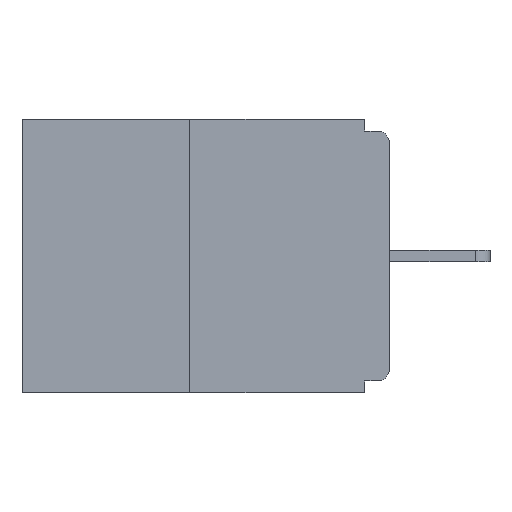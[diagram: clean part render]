
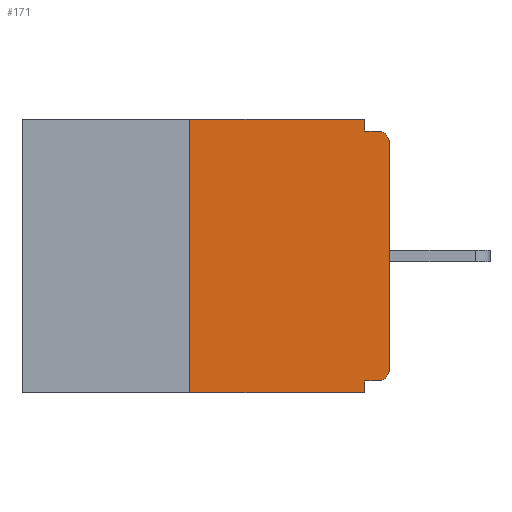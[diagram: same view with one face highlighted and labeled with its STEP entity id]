
A CAD part, left-side view. The second image highlights one B-rep face of the part: STEP entity #171.
In plain terms, the highlighted planar face has unit normal (-1, 0, 0).
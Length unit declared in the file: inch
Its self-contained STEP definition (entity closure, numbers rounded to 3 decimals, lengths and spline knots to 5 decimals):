
#47 = LINE ( 'NONE', #8881, #184 ) ;
#171 = ADVANCED_FACE ( 'NONE', ( #5599 ), #9420, .F. ) ;
#184 = VECTOR ( 'NONE', #10004, 39.37008 ) ;
#208 = EDGE_LOOP ( 'NONE', ( #5698, #8267, #6809, #2005, #5004, #4172, #3948, #3840, #4749, #7733 ) ) ;
#215 = CARTESIAN_POINT ( 'NONE',  ( 0., 0.46, -0.343 ) ) ;
#299 = VERTEX_POINT ( 'NONE', #7699 ) ;
#436 = AXIS2_PLACEMENT_3D ( 'NONE', #7407, #6733, #6550 ) ;
#534 = VECTOR ( 'NONE', #6665, 39.37008 ) ;
#879 = LINE ( 'NONE', #5942, #534 ) ;
#942 = CARTESIAN_POINT ( 'NONE',  ( 0., 0.031, -0.015 ) ) ;
#998 = VERTEX_POINT ( 'NONE', #942 ) ;
#1353 = EDGE_CURVE ( 'NONE', #2045, #8101, #3386, .T. ) ;
#1361 = CARTESIAN_POINT ( 'NONE',  ( 0., 0., -0.328 ) ) ;
#1407 = EDGE_CURVE ( 'NONE', #2045, #6537, #3336, .T. ) ;
#1527 = EDGE_CURVE ( 'NONE', #3534, #6537, #2998, .T. ) ;
#1554 = EDGE_CURVE ( 'NONE', #5897, #3534, #2892, .T. ) ;
#1609 = EDGE_CURVE ( 'NONE', #8135, #998, #2805, .T. ) ;
#2005 = ORIENTED_EDGE ( 'NONE', *, *, #1527, .F. ) ;
#2045 = VERTEX_POINT ( 'NONE', #5724 ) ;
#2105 = CARTESIAN_POINT ( 'NONE',  ( 0., 0., -0.015 ) ) ;
#2471 = EDGE_CURVE ( 'NONE', #8101, #8135, #47, .T. ) ;
#2760 = VECTOR ( 'NONE', #3348, 39.37008 ) ;
#2804 = DIRECTION ( 'NONE',  ( 0., 0., 1. ) ) ;
#2805 = LINE ( 'NONE', #10197, #2760 ) ;
#2863 = VECTOR ( 'NONE', #9930, 39.37008 ) ;
#2892 = LINE ( 'NONE', #1361, #2863 ) ;
#2925 = DIRECTION ( 'NONE',  ( 0., -1., 0. ) ) ;
#2951 = VECTOR ( 'NONE', #5788, 39.37008 ) ;
#2992 = CARTESIAN_POINT ( 'NONE',  ( 0., 0.25, 0. ) ) ;
#2998 = LINE ( 'NONE', #4763, #2951 ) ;
#3192 = AXIS2_PLACEMENT_3D ( 'NONE', #7427, #7318, #7304 ) ;
#3228 = VECTOR ( 'NONE', #2925, 39.37008 ) ;
#3336 = LINE ( 'NONE', #215, #3228 ) ;
#3348 = DIRECTION ( 'NONE',  ( 0., 0., -1. ) ) ;
#3366 = VECTOR ( 'NONE', #2804, 39.37008 ) ;
#3386 = LINE ( 'NONE', #2992, #3366 ) ;
#3403 = DIRECTION ( 'NONE',  ( -1., 0., 0. ) ) ;
#3534 = VERTEX_POINT ( 'NONE', #6160 ) ;
#3840 = ORIENTED_EDGE ( 'NONE', *, *, #5633, .T. ) ;
#3948 = ORIENTED_EDGE ( 'NONE', *, *, #9429, .T. ) ;
#3957 = CARTESIAN_POINT ( 'NONE',  ( 0., 0., -0.313 ) ) ;
#4172 = ORIENTED_EDGE ( 'NONE', *, *, #4719, .T. ) ;
#4719 = EDGE_CURVE ( 'NONE', #5897, #8591, #6618, .T. ) ;
#4749 = ORIENTED_EDGE ( 'NONE', *, *, #5171, .F. ) ;
#4763 = CARTESIAN_POINT ( 'NONE',  ( 0., 0.031, -0.343 ) ) ;
#5004 = ORIENTED_EDGE ( 'NONE', *, *, #1554, .F. ) ;
#5067 = DIRECTION ( 'NONE',  ( 0., -1., 0. ) ) ;
#5171 = EDGE_CURVE ( 'NONE', #998, #299, #7346, .T. ) ;
#5196 = VECTOR ( 'NONE', #5067, 39.37008 ) ;
#5599 = FACE_OUTER_BOUND ( 'NONE', #208, .T. ) ;
#5633 = EDGE_CURVE ( 'NONE', #8870, #299, #7892, .T. ) ;
#5698 = ORIENTED_EDGE ( 'NONE', *, *, #2471, .F. ) ;
#5724 = CARTESIAN_POINT ( 'NONE',  ( 0., 0.25, -0.343 ) ) ;
#5788 = DIRECTION ( 'NONE',  ( 0., 0., -1. ) ) ;
#5897 = VERTEX_POINT ( 'NONE', #9774 ) ;
#5942 = CARTESIAN_POINT ( 'NONE',  ( 0., 0., 0. ) ) ;
#6160 = CARTESIAN_POINT ( 'NONE',  ( 0., 0.031, -0.328 ) ) ;
#6537 = VERTEX_POINT ( 'NONE', #9851 ) ;
#6550 = DIRECTION ( 'NONE',  ( 0., 0., -1. ) ) ;
#6618 = CIRCLE ( 'NONE', #3192, 0.015 ) ;
#6665 = DIRECTION ( 'NONE',  ( 0., 0., 1. ) ) ;
#6733 = DIRECTION ( 'NONE',  ( 1., 0., 0. ) ) ;
#6809 = ORIENTED_EDGE ( 'NONE', *, *, #1407, .T. ) ;
#7304 = DIRECTION ( 'NONE',  ( 0., 0., -1. ) ) ;
#7318 = DIRECTION ( 'NONE',  ( -1., 0., 0. ) ) ;
#7346 = LINE ( 'NONE', #2105, #5196 ) ;
#7407 = CARTESIAN_POINT ( 'NONE',  ( 0., 0.46, 0. ) ) ;
#7427 = CARTESIAN_POINT ( 'NONE',  ( 0., 0.015, -0.313 ) ) ;
#7699 = CARTESIAN_POINT ( 'NONE',  ( 0., 0.015, -0.015 ) ) ;
#7733 = ORIENTED_EDGE ( 'NONE', *, *, #1609, .F. ) ;
#7888 = DIRECTION ( 'NONE',  ( 0., 0., -1. ) ) ;
#7892 = CIRCLE ( 'NONE', #9378, 0.015 ) ;
#8101 = VERTEX_POINT ( 'NONE', #9097 ) ;
#8135 = VERTEX_POINT ( 'NONE', #9319 ) ;
#8267 = ORIENTED_EDGE ( 'NONE', *, *, #1353, .F. ) ;
#8591 = VERTEX_POINT ( 'NONE', #3957 ) ;
#8635 = CARTESIAN_POINT ( 'NONE',  ( 0., 0.015, -0.03 ) ) ;
#8870 = VERTEX_POINT ( 'NONE', #9699 ) ;
#8881 = CARTESIAN_POINT ( 'NONE',  ( 0., 0.46, 0. ) ) ;
#9097 = CARTESIAN_POINT ( 'NONE',  ( 0., 0.25, 0. ) ) ;
#9319 = CARTESIAN_POINT ( 'NONE',  ( 0., 0.031, 0. ) ) ;
#9378 = AXIS2_PLACEMENT_3D ( 'NONE', #8635, #3403, #7888 ) ;
#9420 = PLANE ( 'NONE',  #436 ) ;
#9429 = EDGE_CURVE ( 'NONE', #8591, #8870, #879, .T. ) ;
#9699 = CARTESIAN_POINT ( 'NONE',  ( 0., 0., -0.03 ) ) ;
#9774 = CARTESIAN_POINT ( 'NONE',  ( 0., 0.015, -0.328 ) ) ;
#9851 = CARTESIAN_POINT ( 'NONE',  ( 0., 0.031, -0.343 ) ) ;
#9930 = DIRECTION ( 'NONE',  ( 0., 1., 0. ) ) ;
#10004 = DIRECTION ( 'NONE',  ( 0., -1., 0. ) ) ;
#10197 = CARTESIAN_POINT ( 'NONE',  ( 0., 0.031, 0. ) ) ;
